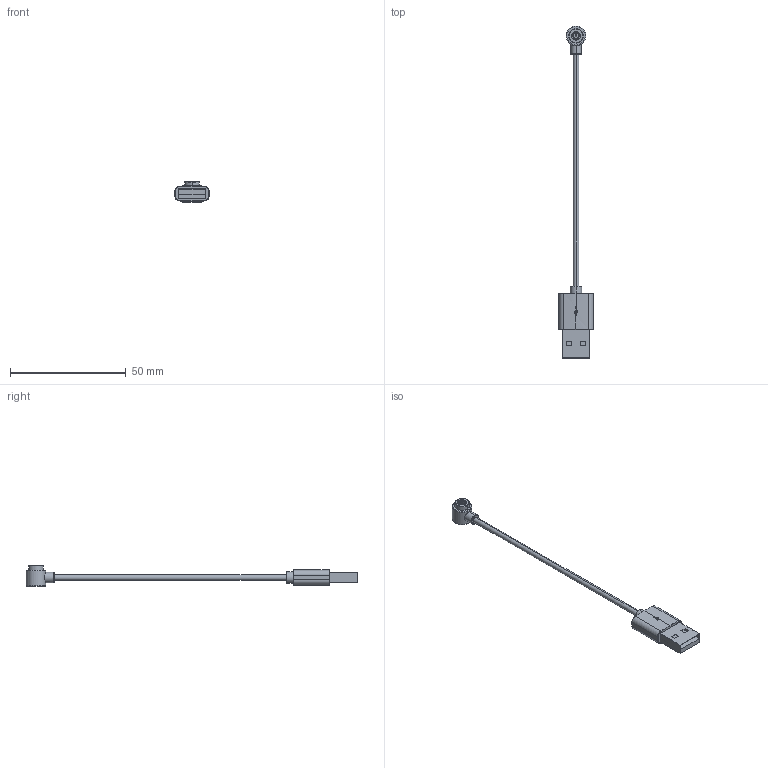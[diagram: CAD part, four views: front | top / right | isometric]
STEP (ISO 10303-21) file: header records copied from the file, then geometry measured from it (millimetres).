
FILE_DESCRIPTION (( 'STEP AP203' ), '1' );
FILE_NAME ('687-B02C2A000J00.STEP', '2023-02-03T17:06:11', ( 'Magnum' ), ( '' ), 'SwSTEP 2.0', 'SolidWorks 2020', '' );
FILE_SCHEMA (( 'CONFIG_CONTROL_DESIGN' ));
Length unit declared in the file: millimetre
Products named in the file (1): 687-B02C2A000J00
Bounding box: 14.8 x 143.25 x 9 mm (x, y, z)
Volume: 2852.2 mm3; surface area: 3001.2 mm2
Topology: 1 solids, 6 shells, 152 faces, 372 edges, 241 vertices
Faces by surface type: plane 68, cylinder 50, torus 25, bspline 5, cone 2, sphere 2
Entity records: 4909 total; most frequent: CARTESIAN_POINT 1194, DIRECTION 781, ORIENTED_EDGE 740, EDGE_CURVE 370, AXIS2_PLACEMENT_3D 313, VERTEX_POINT 241, EDGE_LOOP 177, CIRCLE 165
